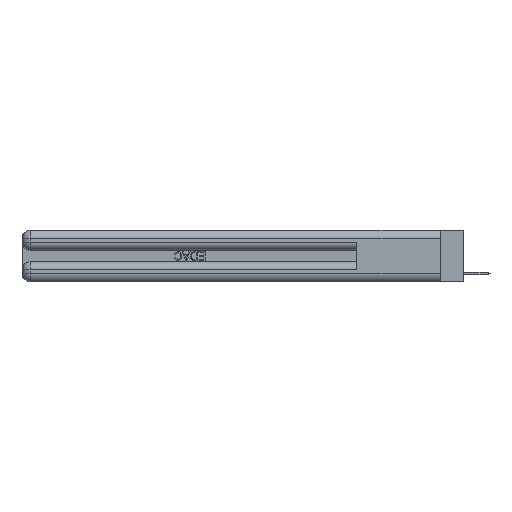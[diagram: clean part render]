
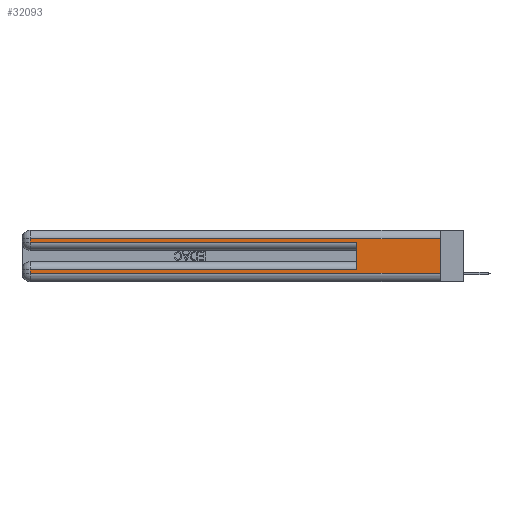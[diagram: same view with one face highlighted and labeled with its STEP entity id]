
A CAD part, left-side view. The second image highlights one B-rep face of the part: STEP entity #32093.
In plain terms, the highlighted planar face has unit normal (-1, 0, 0).
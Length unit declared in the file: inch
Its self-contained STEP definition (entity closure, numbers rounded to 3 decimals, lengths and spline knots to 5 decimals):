
#271 = EDGE_CURVE ( 'NONE', #16587, #33735, #12835, .T. ) ;
#458 = ORIENTED_EDGE ( 'NONE', *, *, #5526, .T. ) ;
#508 = VECTOR ( 'NONE', #13785, 39.37008 ) ;
#730 = CARTESIAN_POINT ( 'NONE',  ( 0., 0., 0.37 ) ) ;
#737 = DIRECTION ( 'NONE',  ( 0., 0., -1. ) ) ;
#947 = LINE ( 'NONE', #730, #508 ) ;
#3459 = PLANE ( 'NONE',  #12424 ) ;
#3589 = CARTESIAN_POINT ( 'NONE',  ( 0., 0., 0.285 ) ) ;
#4037 = VERTEX_POINT ( 'NONE', #30277 ) ;
#4263 = EDGE_LOOP ( 'NONE', ( #23188, #7028, #24627, #6231, #31095, #458, #34038, #27474 ) ) ;
#4713 = CARTESIAN_POINT ( 'NONE',  ( 0., 2.94, 0.37 ) ) ;
#5526 = EDGE_CURVE ( 'NONE', #26458, #22682, #22941, .T. ) ;
#5588 = CARTESIAN_POINT ( 'NONE',  ( 0., 0., 0.31 ) ) ;
#5654 = DIRECTION ( 'NONE',  ( 0., 0., 1. ) ) ;
#5659 = VECTOR ( 'NONE', #5654, 39.37008 ) ;
#5833 = EDGE_CURVE ( 'NONE', #16587, #30696, #947, .T. ) ;
#6053 = DIRECTION ( 'NONE',  ( 0., 0., -1. ) ) ;
#6231 = ORIENTED_EDGE ( 'NONE', *, *, #9942, .T. ) ;
#6350 = CARTESIAN_POINT ( 'NONE',  ( 0., 0., 0.06 ) ) ;
#6538 = DIRECTION ( 'NONE',  ( 0., -1., 0. ) ) ;
#6883 = VECTOR ( 'NONE', #7527, 39.37008 ) ;
#7028 = ORIENTED_EDGE ( 'NONE', *, *, #271, .T. ) ;
#7527 = DIRECTION ( 'NONE',  ( 0., 0., -1. ) ) ;
#7529 = LINE ( 'NONE', #6350, #13826 ) ;
#7668 = VECTOR ( 'NONE', #737, 39.37008 ) ;
#8691 = CARTESIAN_POINT ( 'NONE',  ( 0., 0., 0.085 ) ) ;
#9434 = CARTESIAN_POINT ( 'NONE',  ( 0., 2.94, 0.31 ) ) ;
#9942 = EDGE_CURVE ( 'NONE', #16346, #32069, #25182, .T. ) ;
#10493 = CARTESIAN_POINT ( 'NONE',  ( 0., 0., 0.31 ) ) ;
#10971 = EDGE_CURVE ( 'NONE', #33735, #16346, #14837, .T. ) ;
#12424 = AXIS2_PLACEMENT_3D ( 'NONE', #22224, #27886, #6053 ) ;
#12835 = LINE ( 'NONE', #5588, #33522 ) ;
#13785 = DIRECTION ( 'NONE',  ( 0., 0., -1. ) ) ;
#13826 = VECTOR ( 'NONE', #25250, 39.37008 ) ;
#14560 = CARTESIAN_POINT ( 'NONE',  ( 0., 0., 0.06 ) ) ;
#14837 = LINE ( 'NONE', #27636, #7668 ) ;
#16346 = VERTEX_POINT ( 'NONE', #28708 ) ;
#16587 = VERTEX_POINT ( 'NONE', #10493 ) ;
#17138 = DIRECTION ( 'NONE',  ( 0., 1., 0. ) ) ;
#18650 = EDGE_CURVE ( 'NONE', #26458, #32069, #30965, .T. ) ;
#21919 = EDGE_CURVE ( 'NONE', #4037, #30696, #7529, .T. ) ;
#22224 = CARTESIAN_POINT ( 'NONE',  ( 0., 0., 0.37 ) ) ;
#22579 = CARTESIAN_POINT ( 'NONE',  ( 0., 0.6, 0.285 ) ) ;
#22682 = VERTEX_POINT ( 'NONE', #33713 ) ;
#22941 = LINE ( 'NONE', #8691, #33016 ) ;
#23188 = ORIENTED_EDGE ( 'NONE', *, *, #5833, .F. ) ;
#23734 = EDGE_CURVE ( 'NONE', #22682, #4037, #27142, .T. ) ;
#24627 = ORIENTED_EDGE ( 'NONE', *, *, #10971, .T. ) ;
#24752 = VECTOR ( 'NONE', #6538, 39.37008 ) ;
#25182 = LINE ( 'NONE', #3589, #24752 ) ;
#25250 = DIRECTION ( 'NONE',  ( 0., -1., 0. ) ) ;
#26458 = VERTEX_POINT ( 'NONE', #31576 ) ;
#27142 = LINE ( 'NONE', #4713, #6883 ) ;
#27337 = FACE_OUTER_BOUND ( 'NONE', #4263, .T. ) ;
#27474 = ORIENTED_EDGE ( 'NONE', *, *, #21919, .T. ) ;
#27636 = CARTESIAN_POINT ( 'NONE',  ( 0., 2.94, 0.37 ) ) ;
#27886 = DIRECTION ( 'NONE',  ( 1., 0., 0. ) ) ;
#28708 = CARTESIAN_POINT ( 'NONE',  ( 0., 2.94, 0.285 ) ) ;
#30213 = DIRECTION ( 'NONE',  ( 0., 1., 0. ) ) ;
#30277 = CARTESIAN_POINT ( 'NONE',  ( 0., 2.94, 0.06 ) ) ;
#30696 = VERTEX_POINT ( 'NONE', #14560 ) ;
#30965 = LINE ( 'NONE', #32522, #5659 ) ;
#31095 = ORIENTED_EDGE ( 'NONE', *, *, #18650, .F. ) ;
#31576 = CARTESIAN_POINT ( 'NONE',  ( 0., 0.6, 0.085 ) ) ;
#32069 = VERTEX_POINT ( 'NONE', #22579 ) ;
#32093 = ADVANCED_FACE ( 'NONE', ( #27337 ), #3459, .F. ) ;
#32522 = CARTESIAN_POINT ( 'NONE',  ( 0., 0.6, 0.145 ) ) ;
#33016 = VECTOR ( 'NONE', #17138, 39.37008 ) ;
#33522 = VECTOR ( 'NONE', #30213, 39.37008 ) ;
#33713 = CARTESIAN_POINT ( 'NONE',  ( 0., 2.94, 0.085 ) ) ;
#33735 = VERTEX_POINT ( 'NONE', #9434 ) ;
#34038 = ORIENTED_EDGE ( 'NONE', *, *, #23734, .T. ) ;
